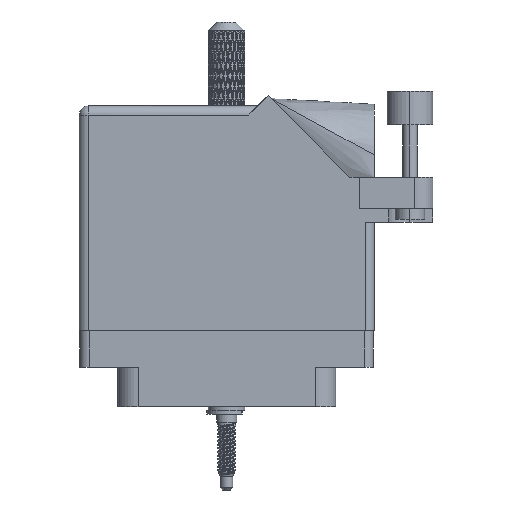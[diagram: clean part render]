
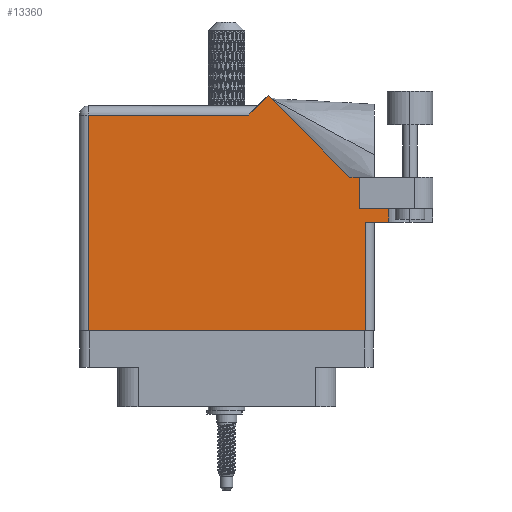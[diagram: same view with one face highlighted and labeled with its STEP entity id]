
A CAD part, front view. The second image highlights one B-rep face of the part: STEP entity #13360.
In plain terms, the highlighted face is planar.
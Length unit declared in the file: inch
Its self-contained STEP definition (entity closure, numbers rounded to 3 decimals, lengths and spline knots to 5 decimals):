
#236 = VECTOR ( 'NONE', #2475, 39.37008 ) ;
#460 = VERTEX_POINT ( 'NONE', #45939 ) ;
#2332 = EDGE_CURVE ( 'NONE', #80398, #460, #83484, .T. ) ;
#2475 = DIRECTION ( 'NONE',  ( 0., -1., 0. ) ) ;
#3405 = LINE ( 'NONE', #79885, #63585 ) ;
#4382 = EDGE_CURVE ( 'NONE', #58919, #80398, #70407, .T. ) ;
#5234 = CARTESIAN_POINT ( 'NONE',  ( 0.905, 0.731, 0.455 ) ) ;
#6665 = DIRECTION ( 'NONE',  ( 0., -1., 0. ) ) ;
#7114 = CARTESIAN_POINT ( 'NONE',  ( 0.905, 0.731, 0.455 ) ) ;
#7334 = LINE ( 'NONE', #44075, #72680 ) ;
#7512 = DIRECTION ( 'NONE',  ( 0., 0., -1. ) ) ;
#9239 = VERTEX_POINT ( 'NONE', #33104 ) ;
#10498 = EDGE_CURVE ( 'NONE', #83074, #81161, #36622, .T. ) ;
#11219 = DIRECTION ( 'NONE',  ( -1., 0., 0. ) ) ;
#12250 = CARTESIAN_POINT ( 'NONE',  ( 0.905, 0.731, 0.455 ) ) ;
#13360 = ADVANCED_FACE ( 'NONE', ( #36433 ), #80977, .F. ) ;
#16461 = EDGE_CURVE ( 'NONE', #58919, #100035, #88610, .T. ) ;
#18952 = CARTESIAN_POINT ( 'NONE',  ( 0.943, 0.637, 0.455 ) ) ;
#20742 = DIRECTION ( 'NONE',  ( 0., 1., 0. ) ) ;
#21252 = VERTEX_POINT ( 'NONE', #91420 ) ;
#21444 = VECTOR ( 'NONE', #26567, 39.37008 ) ;
#21817 = CARTESIAN_POINT ( 'NONE',  ( -0.943, -0.1, 0.455 ) ) ;
#22264 = DIRECTION ( 'NONE',  ( -0.707, -0.707, 0. ) ) ;
#22267 = ORIENTED_EDGE ( 'NONE', *, *, #27157, .T. ) ;
#22580 = VECTOR ( 'NONE', #38049, 39.37008 ) ;
#22735 = LINE ( 'NONE', #26200, #21444 ) ;
#23087 = VECTOR ( 'NONE', #30852, 39.37008 ) ;
#23881 = ORIENTED_EDGE ( 'NONE', *, *, #2332, .F. ) ;
#26200 = CARTESIAN_POINT ( 'NONE',  ( 0.943, 0.637, 0.455 ) ) ;
#26567 = DIRECTION ( 'NONE',  ( 0., 1., 0. ) ) ;
#26987 = VECTOR ( 'NONE', #6665, 39.37008 ) ;
#27157 = EDGE_CURVE ( 'NONE', #21252, #93262, #22735, .T. ) ;
#28295 = DIRECTION ( 'NONE',  ( -0.707, 0.707, 0. ) ) ;
#30394 = LINE ( 'NONE', #60270, #80285 ) ;
#30852 = DIRECTION ( 'NONE',  ( 1., 0., 0. ) ) ;
#31674 = ORIENTED_EDGE ( 'NONE', *, *, #40554, .T. ) ;
#31939 = DIRECTION ( 'NONE',  ( -1., 0., 0. ) ) ;
#33104 = CARTESIAN_POINT ( 'NONE',  ( -0.943, -0.1, 0.455 ) ) ;
#33296 = CARTESIAN_POINT ( 'NONE',  ( -0.943, 1.368, 0.455 ) ) ;
#35695 = ORIENTED_EDGE ( 'NONE', *, *, #64388, .T. ) ;
#36433 = FACE_OUTER_BOUND ( 'NONE', #77664, .T. ) ;
#36622 = LINE ( 'NONE', #60425, #52006 ) ;
#38049 = DIRECTION ( 'NONE',  ( -1., 0., 0. ) ) ;
#39000 = VERTEX_POINT ( 'NONE', #33296 ) ;
#40554 = EDGE_CURVE ( 'NONE', #100035, #83074, #30394, .T. ) ;
#42605 = CARTESIAN_POINT ( 'NONE',  ( 0.28271, 1.50071, 0.455 ) ) ;
#44075 = CARTESIAN_POINT ( 'NONE',  ( -1.005, -0.1, 0.455 ) ) ;
#44887 = ORIENTED_EDGE ( 'NONE', *, *, #47293, .T. ) ;
#45907 = CARTESIAN_POINT ( 'NONE',  ( -1.005, 1.368, 0.455 ) ) ;
#45939 = CARTESIAN_POINT ( 'NONE',  ( 1.1065, 0.637, 0.455 ) ) ;
#47293 = EDGE_CURVE ( 'NONE', #81161, #50363, #103888, .T. ) ;
#50363 = VERTEX_POINT ( 'NONE', #86291 ) ;
#51589 = CARTESIAN_POINT ( 'NONE',  ( 1.1065, 1.06177, 0.455 ) ) ;
#52006 = VECTOR ( 'NONE', #28295, 39.37008 ) ;
#56463 = VECTOR ( 'NONE', #22264, 39.37008 ) ;
#58919 = VERTEX_POINT ( 'NONE', #12250 ) ;
#60270 = CARTESIAN_POINT ( 'NONE',  ( 1.405, 0.944, 0.455 ) ) ;
#60425 = CARTESIAN_POINT ( 'NONE',  ( 0.83942, 0.944, 0.455 ) ) ;
#63585 = VECTOR ( 'NONE', #80601, 39.37008 ) ;
#64388 = EDGE_CURVE ( 'NONE', #50363, #39000, #98210, .T. ) ;
#70407 = LINE ( 'NONE', #7114, #23087 ) ;
#70532 = LINE ( 'NONE', #21817, #26987 ) ;
#72680 = VECTOR ( 'NONE', #100336, 39.37008 ) ;
#74343 = EDGE_CURVE ( 'NONE', #39000, #9239, #70532, .T. ) ;
#76347 = CARTESIAN_POINT ( 'NONE',  ( 0.905, 0.944, 0.455 ) ) ;
#76704 = ORIENTED_EDGE ( 'NONE', *, *, #4382, .F. ) ;
#76761 = EDGE_CURVE ( 'NONE', #9239, #21252, #7334, .T. ) ;
#77664 = EDGE_LOOP ( 'NONE', ( #94880, #22267, #96100, #23881, #76704, #91830, #31674, #89485, #44887, #35695, #80908 ) ) ;
#79804 = AXIS2_PLACEMENT_3D ( 'NONE', #98169, #7512, #31939 ) ;
#79885 = CARTESIAN_POINT ( 'NONE',  ( 1.005, 0.637, 0.455 ) ) ;
#80285 = VECTOR ( 'NONE', #11219, 39.37008 ) ;
#80398 = VERTEX_POINT ( 'NONE', #100523 ) ;
#80601 = DIRECTION ( 'NONE',  ( 1., 0., 0. ) ) ;
#80908 = ORIENTED_EDGE ( 'NONE', *, *, #74343, .T. ) ;
#80977 = PLANE ( 'NONE',  #79804 ) ;
#81161 = VERTEX_POINT ( 'NONE', #42605 ) ;
#83074 = VERTEX_POINT ( 'NONE', #102063 ) ;
#83484 = LINE ( 'NONE', #51589, #236 ) ;
#86291 = CARTESIAN_POINT ( 'NONE',  ( 0.15, 1.368, 0.455 ) ) ;
#88610 = LINE ( 'NONE', #5234, #97575 ) ;
#89485 = ORIENTED_EDGE ( 'NONE', *, *, #10498, .T. ) ;
#91420 = CARTESIAN_POINT ( 'NONE',  ( 0.943, -0.1, 0.455 ) ) ;
#91830 = ORIENTED_EDGE ( 'NONE', *, *, #16461, .T. ) ;
#93262 = VERTEX_POINT ( 'NONE', #18952 ) ;
#94880 = ORIENTED_EDGE ( 'NONE', *, *, #76761, .T. ) ;
#95371 = CARTESIAN_POINT ( 'NONE',  ( 0.212, 1.43, 0.455 ) ) ;
#96100 = ORIENTED_EDGE ( 'NONE', *, *, #105015, .T. ) ;
#97575 = VECTOR ( 'NONE', #20742, 39.37008 ) ;
#98169 = CARTESIAN_POINT ( 'NONE',  ( -1.005, 1.43, 0.455 ) ) ;
#98210 = LINE ( 'NONE', #45907, #22580 ) ;
#100035 = VERTEX_POINT ( 'NONE', #76347 ) ;
#100336 = DIRECTION ( 'NONE',  ( 1., 0., 0. ) ) ;
#100523 = CARTESIAN_POINT ( 'NONE',  ( 1.1065, 0.731, 0.455 ) ) ;
#102063 = CARTESIAN_POINT ( 'NONE',  ( 0.83942, 0.944, 0.455 ) ) ;
#103888 = LINE ( 'NONE', #95371, #56463 ) ;
#105015 = EDGE_CURVE ( 'NONE', #93262, #460, #3405, .T. ) ;
